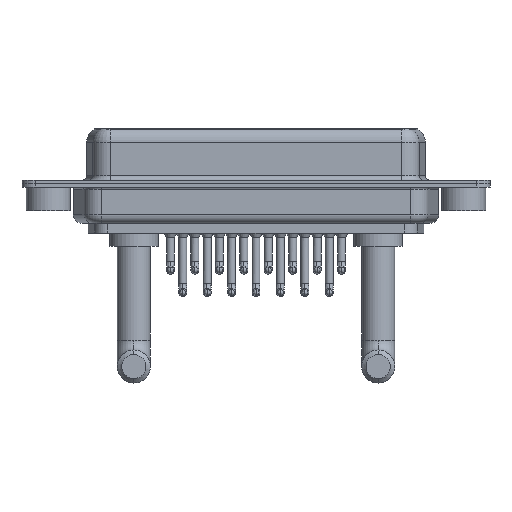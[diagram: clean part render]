
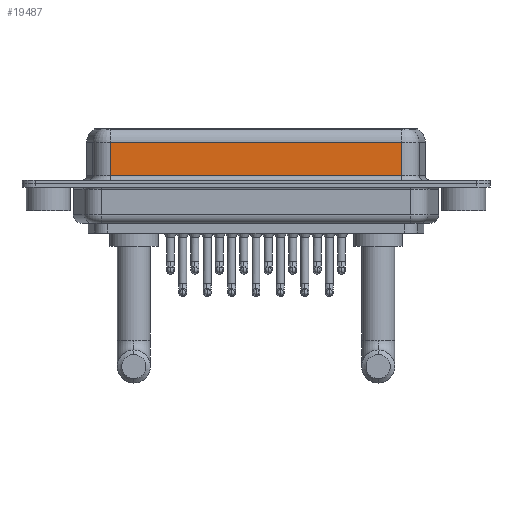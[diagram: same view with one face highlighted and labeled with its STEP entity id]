
A CAD part, front view. The second image highlights one B-rep face of the part: STEP entity #19487.
In plain terms, the highlighted planar face has unit normal (0, -1, 0).
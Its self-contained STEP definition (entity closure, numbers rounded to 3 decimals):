
#282 = EDGE_CURVE ( 'NONE', #19517, #6666, #13844, .T. ) ;
#992 = LINE ( 'NONE', #5544, #15979 ) ;
#2070 = PLANE ( 'NONE',  #10553 ) ;
#3451 = FACE_OUTER_BOUND ( 'NONE', #15366, .T. ) ;
#4343 = VERTEX_POINT ( 'NONE', #6655 ) ;
#4365 = DIRECTION ( 'NONE',  ( 0., 0., -1. ) ) ;
#5544 = CARTESIAN_POINT ( 'NONE',  ( 7.013, -3.95, 6.4 ) ) ;
#6402 = DIRECTION ( 'NONE',  ( 0., 1., 0. ) ) ;
#6441 = VECTOR ( 'NONE', #11342, 1000. ) ;
#6503 = DIRECTION ( 'NONE',  ( 0., 0., 1. ) ) ;
#6655 = CARTESIAN_POINT ( 'NONE',  ( 7.013, -3.95, 0.9 ) ) ;
#6666 = VERTEX_POINT ( 'NONE', #13349 ) ;
#7270 = CARTESIAN_POINT ( 'NONE',  ( 40.037, -3.95, 0.9 ) ) ;
#8247 = VERTEX_POINT ( 'NONE', #7270 ) ;
#8325 = DIRECTION ( 'NONE',  ( 1., 0., 0. ) ) ;
#8514 = VECTOR ( 'NONE', #19180, 1000. ) ;
#10553 = AXIS2_PLACEMENT_3D ( 'NONE', #16401, #6402, #6503 ) ;
#10697 = CARTESIAN_POINT ( 'NONE',  ( 40.037, -3.95, 4.65 ) ) ;
#11342 = DIRECTION ( 'NONE',  ( 0., 0., -1. ) ) ;
#11435 = ORIENTED_EDGE ( 'NONE', *, *, #282, .T. ) ;
#12369 = ORIENTED_EDGE ( 'NONE', *, *, #15171, .T. ) ;
#12598 = LINE ( 'NONE', #19229, #6441 ) ;
#13349 = CARTESIAN_POINT ( 'NONE',  ( 7.013, -3.95, 4.65 ) ) ;
#13791 = ORIENTED_EDGE ( 'NONE', *, *, #20647, .T. ) ;
#13844 = LINE ( 'NONE', #10697, #8514 ) ;
#14221 = ORIENTED_EDGE ( 'NONE', *, *, #15535, .F. ) ;
#14708 = CARTESIAN_POINT ( 'NONE',  ( 40.037, -3.95, 4.65 ) ) ;
#15171 = EDGE_CURVE ( 'NONE', #4343, #8247, #17882, .T. ) ;
#15366 = EDGE_LOOP ( 'NONE', ( #14221, #11435, #13791, #12369 ) ) ;
#15535 = EDGE_CURVE ( 'NONE', #19517, #8247, #12598, .T. ) ;
#15979 = VECTOR ( 'NONE', #4365, 1000. ) ;
#16401 = CARTESIAN_POINT ( 'NONE',  ( 40.037, -3.95, 6.4 ) ) ;
#17882 = LINE ( 'NONE', #19363, #20196 ) ;
#19180 = DIRECTION ( 'NONE',  ( -1., 0., 0. ) ) ;
#19229 = CARTESIAN_POINT ( 'NONE',  ( 40.037, -3.95, 6.4 ) ) ;
#19363 = CARTESIAN_POINT ( 'NONE',  ( 40.037, -3.95, 0.9 ) ) ;
#19487 = ADVANCED_FACE ( 'NONE', ( #3451 ), #2070, .F. ) ;
#19517 = VERTEX_POINT ( 'NONE', #14708 ) ;
#20196 = VECTOR ( 'NONE', #8325, 1000. ) ;
#20647 = EDGE_CURVE ( 'NONE', #6666, #4343, #992, .T. ) ;
